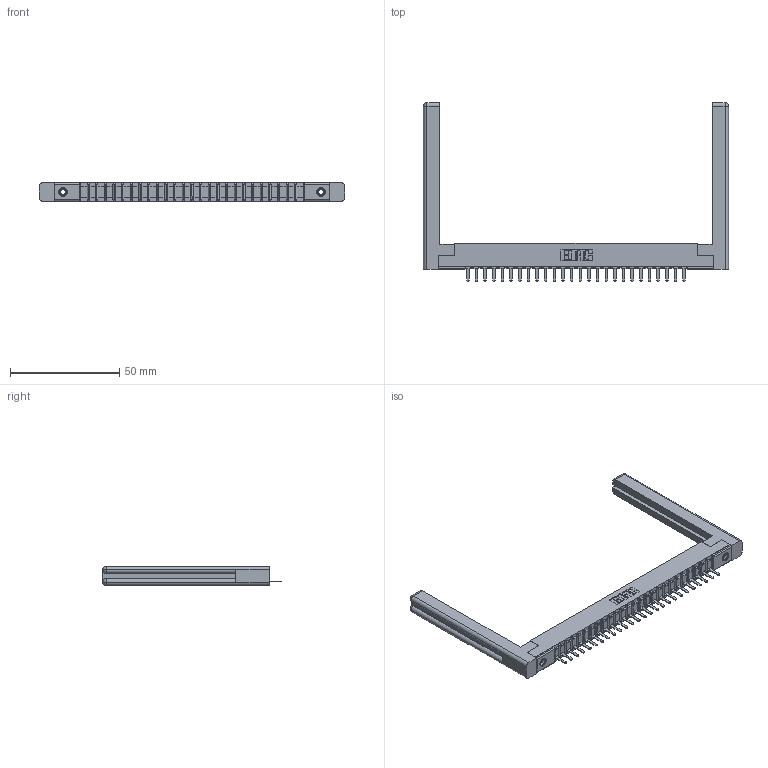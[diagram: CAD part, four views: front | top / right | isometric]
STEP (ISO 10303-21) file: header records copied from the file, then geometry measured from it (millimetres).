
FILE_DESCRIPTION (( 'STEP AP203' ), '1' );
FILE_NAME ('357-026-421-158.STEP', '2020-10-01T17:27:27', ( '' ), ( '' ), 'SwSTEP 2.0', 'SolidWorks 2020', '' );
FILE_SCHEMA (( 'CONFIG_CONTROL_DESIGN' ));
Length unit declared in the file: inch
Products named in the file (5): 307-220-058; 345-250-001_345-250-001-102; 307 Part_.156 Dia Mounting Holes; 307-290-002_521; 357-026-421-158
Assembly tree (31 placements, depth 2):
  357-026-421-158
    307 Part_.156 Dia Mounting Holes
    307-290-002_521  x26
    307-220-058  x2
    345-250-001_345-250-001-102  x2
Bounding box: 139.65 x 81.74 x 8.71 mm (x, y, z)
Volume: 16901.3 mm3; surface area: 22037.4 mm2
Topology: 31 solids, 31 shells, 2211 faces, 6709 edges, 4386 vertices
Faces by surface type: plane 1324, cylinder 809, sphere 54, torus 12, cone 12
Entity records: 27613 total; most frequent: CARTESIAN_POINT 4663, ORIENTED_EDGE 4592, DIRECTION 4498, EDGE_CURVE 2296, LINE 1748, VECTOR 1748, VERTEX_POINT 1486, AXIS2_PLACEMENT_3D 1375
